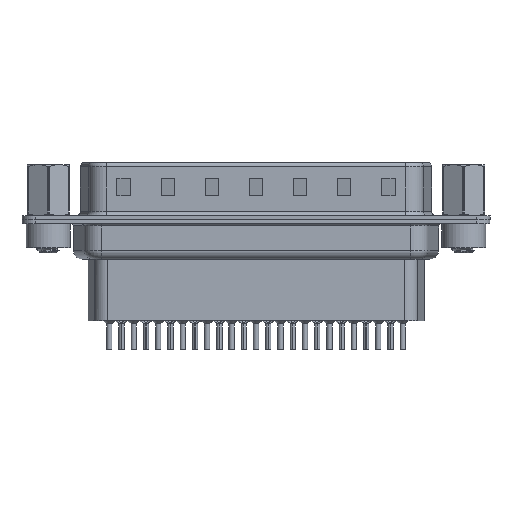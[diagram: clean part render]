
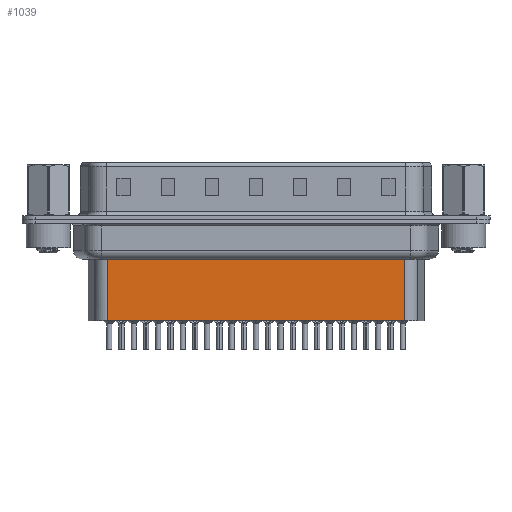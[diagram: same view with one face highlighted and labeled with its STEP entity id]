
A CAD part, front view. The second image highlights one B-rep face of the part: STEP entity #1039.
In plain terms, the highlighted planar face has unit normal (0, -1, 0).
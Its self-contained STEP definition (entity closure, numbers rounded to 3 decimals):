
#665 = CARTESIAN_POINT ( 'NONE',  ( 40.344, -3.5, -11.45 ) ) ;
#872 = VECTOR ( 'NONE', #24548, 1000. ) ;
#1039 = ADVANCED_FACE ( 'NONE', ( #24000 ), #4813, .T. ) ;
#1633 = CARTESIAN_POINT ( 'NONE',  ( 6.706, -3.5, -3.1 ) ) ;
#3944 = ORIENTED_EDGE ( 'NONE', *, *, #27768, .F. ) ;
#4082 = CARTESIAN_POINT ( 'NONE',  ( 40.344, -3.5, -4.097 ) ) ;
#4813 = PLANE ( 'NONE',  #6859 ) ;
#6681 = EDGE_CURVE ( 'NONE', #21376, #12166, #16110, .T. ) ;
#6699 = VECTOR ( 'NONE', #24213, 1000. ) ;
#6839 = DIRECTION ( 'NONE',  ( 1., 0., 0. ) ) ;
#6856 = DIRECTION ( 'NONE',  ( 0., 0., -1. ) ) ;
#6859 = AXIS2_PLACEMENT_3D ( 'NONE', #1633, #6966, #6839 ) ;
#6966 = DIRECTION ( 'NONE',  ( 0., -1., 0. ) ) ;
#8163 = CARTESIAN_POINT ( 'NONE',  ( 6.459, -3.5, -4.097 ) ) ;
#8505 = CARTESIAN_POINT ( 'NONE',  ( 40.344, -3.5, -3.1 ) ) ;
#9923 = LINE ( 'NONE', #25870, #16023 ) ;
#11199 = EDGE_LOOP ( 'NONE', ( #3944, #20476, #15618, #29403 ) ) ;
#12166 = VERTEX_POINT ( 'NONE', #24526 ) ;
#12937 = VERTEX_POINT ( 'NONE', #4082 ) ;
#15618 = ORIENTED_EDGE ( 'NONE', *, *, #6681, .T. ) ;
#16023 = VECTOR ( 'NONE', #28213, 1000. ) ;
#16110 = LINE ( 'NONE', #18353, #21506 ) ;
#17986 = EDGE_CURVE ( 'NONE', #12937, #21376, #25046, .T. ) ;
#18353 = CARTESIAN_POINT ( 'NONE',  ( 6.706, -3.5, -3.1 ) ) ;
#20476 = ORIENTED_EDGE ( 'NONE', *, *, #17986, .T. ) ;
#21376 = VERTEX_POINT ( 'NONE', #22854 ) ;
#21506 = VECTOR ( 'NONE', #6856, 1000. ) ;
#22854 = CARTESIAN_POINT ( 'NONE',  ( 6.706, -3.5, -4.097 ) ) ;
#23908 = EDGE_CURVE ( 'NONE', #25830, #12166, #9923, .T. ) ;
#24000 = FACE_OUTER_BOUND ( 'NONE', #11199, .T. ) ;
#24213 = DIRECTION ( 'NONE',  ( -1., 0., 0. ) ) ;
#24526 = CARTESIAN_POINT ( 'NONE',  ( 6.706, -3.5, -11.45 ) ) ;
#24548 = DIRECTION ( 'NONE',  ( 0., 0., -1. ) ) ;
#25046 = LINE ( 'NONE', #8163, #6699 ) ;
#25830 = VERTEX_POINT ( 'NONE', #665 ) ;
#25870 = CARTESIAN_POINT ( 'NONE',  ( 6.706, -3.5, -11.45 ) ) ;
#27768 = EDGE_CURVE ( 'NONE', #12937, #25830, #29445, .T. ) ;
#28213 = DIRECTION ( 'NONE',  ( -1., 0., 0. ) ) ;
#29403 = ORIENTED_EDGE ( 'NONE', *, *, #23908, .F. ) ;
#29445 = LINE ( 'NONE', #8505, #872 ) ;
